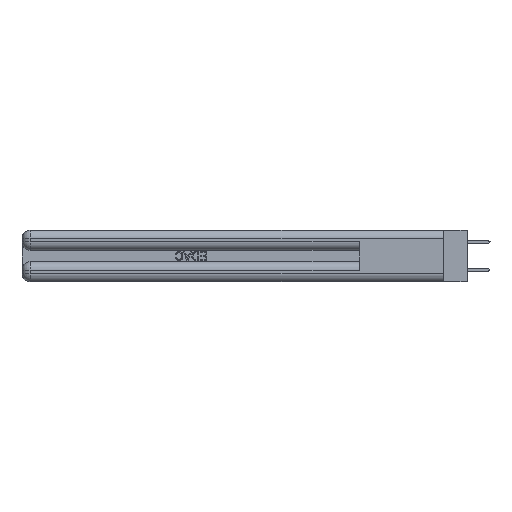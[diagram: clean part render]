
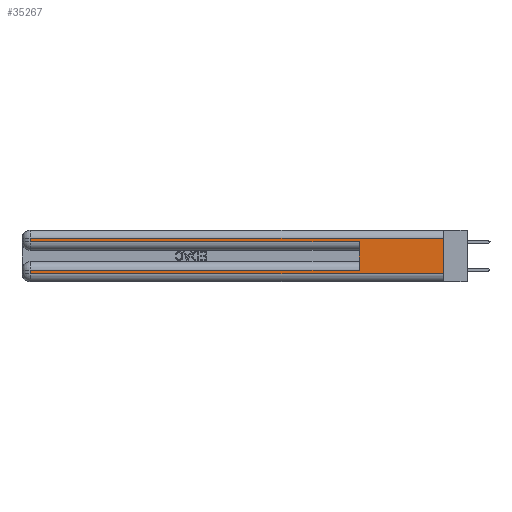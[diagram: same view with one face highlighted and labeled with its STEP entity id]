
A CAD part, left-side view. The second image highlights one B-rep face of the part: STEP entity #35267.
In plain terms, the highlighted planar face has unit normal (-1, 0, 0).
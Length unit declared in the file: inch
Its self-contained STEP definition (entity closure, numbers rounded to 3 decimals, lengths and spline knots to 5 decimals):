
#135 = ORIENTED_EDGE ( 'NONE', *, *, #6868, .T. ) ;
#209 = DIRECTION ( 'NONE',  ( 0., 1., 0. ) ) ;
#289 = CARTESIAN_POINT ( 'NONE',  ( 0., 0., 0.31 ) ) ;
#968 = VECTOR ( 'NONE', #209, 39.37008 ) ;
#1395 = LINE ( 'NONE', #9236, #25498 ) ;
#1719 = LINE ( 'NONE', #32343, #16856 ) ;
#1926 = LINE ( 'NONE', #24377, #968 ) ;
#2803 = VECTOR ( 'NONE', #30012, 39.37008 ) ;
#4164 = CARTESIAN_POINT ( 'NONE',  ( 0., 0., 0.06 ) ) ;
#4578 = CARTESIAN_POINT ( 'NONE',  ( 0., 2.94, 0.31 ) ) ;
#4890 = CARTESIAN_POINT ( 'NONE',  ( 0., 0., 0.37 ) ) ;
#5963 = CARTESIAN_POINT ( 'NONE',  ( 0., 0.6, 0.085 ) ) ;
#6315 = ORIENTED_EDGE ( 'NONE', *, *, #35557, .T. ) ;
#6868 = EDGE_CURVE ( 'NONE', #13591, #37456, #1926, .T. ) ;
#7078 = VECTOR ( 'NONE', #18430, 39.37008 ) ;
#7942 = PLANE ( 'NONE',  #19348 ) ;
#8632 = VECTOR ( 'NONE', #34360, 39.37008 ) ;
#9236 = CARTESIAN_POINT ( 'NONE',  ( 0., 2.94, 0.37 ) ) ;
#9917 = LINE ( 'NONE', #15389, #7078 ) ;
#9957 = FACE_OUTER_BOUND ( 'NONE', #37861, .T. ) ;
#10875 = LINE ( 'NONE', #24101, #2803 ) ;
#10936 = EDGE_CURVE ( 'NONE', #37456, #20333, #11874, .T. ) ;
#10943 = VECTOR ( 'NONE', #12433, 39.37008 ) ;
#11874 = LINE ( 'NONE', #27427, #10943 ) ;
#12265 = DIRECTION ( 'NONE',  ( 0., 0., -1. ) ) ;
#12402 = VECTOR ( 'NONE', #21755, 39.37008 ) ;
#12433 = DIRECTION ( 'NONE',  ( 0., 0., -1. ) ) ;
#12464 = ORIENTED_EDGE ( 'NONE', *, *, #17266, .F. ) ;
#12747 = VERTEX_POINT ( 'NONE', #4578 ) ;
#13591 = VERTEX_POINT ( 'NONE', #5963 ) ;
#14005 = DIRECTION ( 'NONE',  ( 1., 0., 0. ) ) ;
#14352 = ORIENTED_EDGE ( 'NONE', *, *, #27515, .T. ) ;
#14468 = CARTESIAN_POINT ( 'NONE',  ( 0., 2.94, 0.06 ) ) ;
#15389 = CARTESIAN_POINT ( 'NONE',  ( 0., 0., 0.285 ) ) ;
#16207 = ORIENTED_EDGE ( 'NONE', *, *, #10936, .T. ) ;
#16856 = VECTOR ( 'NONE', #29330, 39.37008 ) ;
#17266 = EDGE_CURVE ( 'NONE', #28186, #18667, #28405, .T. ) ;
#18430 = DIRECTION ( 'NONE',  ( 0., -1., 0. ) ) ;
#18501 = LINE ( 'NONE', #31327, #8632 ) ;
#18667 = VERTEX_POINT ( 'NONE', #4164 ) ;
#18722 = CARTESIAN_POINT ( 'NONE',  ( 0., 0., 0.37 ) ) ;
#19348 = AXIS2_PLACEMENT_3D ( 'NONE', #4890, #14005, #35014 ) ;
#20317 = EDGE_CURVE ( 'NONE', #20333, #18667, #1719, .T. ) ;
#20333 = VERTEX_POINT ( 'NONE', #14468 ) ;
#20448 = ORIENTED_EDGE ( 'NONE', *, *, #24747, .T. ) ;
#21755 = DIRECTION ( 'NONE',  ( 0., 0., -1. ) ) ;
#21944 = VERTEX_POINT ( 'NONE', #22452 ) ;
#22452 = CARTESIAN_POINT ( 'NONE',  ( 0., 2.94, 0.285 ) ) ;
#24101 = CARTESIAN_POINT ( 'NONE',  ( 0., 0.6, 0.145 ) ) ;
#24346 = CARTESIAN_POINT ( 'NONE',  ( 0., 2.94, 0.085 ) ) ;
#24377 = CARTESIAN_POINT ( 'NONE',  ( 0., 0., 0.085 ) ) ;
#24747 = EDGE_CURVE ( 'NONE', #28186, #12747, #18501, .T. ) ;
#25498 = VECTOR ( 'NONE', #12265, 39.37008 ) ;
#27413 = EDGE_CURVE ( 'NONE', #13591, #29452, #10875, .T. ) ;
#27427 = CARTESIAN_POINT ( 'NONE',  ( 0., 2.94, 0.37 ) ) ;
#27515 = EDGE_CURVE ( 'NONE', #21944, #29452, #9917, .T. ) ;
#28186 = VERTEX_POINT ( 'NONE', #289 ) ;
#28405 = LINE ( 'NONE', #18722, #12402 ) ;
#29330 = DIRECTION ( 'NONE',  ( 0., -1., 0. ) ) ;
#29452 = VERTEX_POINT ( 'NONE', #37052 ) ;
#30012 = DIRECTION ( 'NONE',  ( 0., 0., 1. ) ) ;
#31269 = ORIENTED_EDGE ( 'NONE', *, *, #27413, .F. ) ;
#31327 = CARTESIAN_POINT ( 'NONE',  ( 0., 0., 0.31 ) ) ;
#32343 = CARTESIAN_POINT ( 'NONE',  ( 0., 0., 0.06 ) ) ;
#34093 = ORIENTED_EDGE ( 'NONE', *, *, #20317, .T. ) ;
#34360 = DIRECTION ( 'NONE',  ( 0., 1., 0. ) ) ;
#35014 = DIRECTION ( 'NONE',  ( 0., 0., -1. ) ) ;
#35267 = ADVANCED_FACE ( 'NONE', ( #9957 ), #7942, .F. ) ;
#35557 = EDGE_CURVE ( 'NONE', #12747, #21944, #1395, .T. ) ;
#37052 = CARTESIAN_POINT ( 'NONE',  ( 0., 0.6, 0.285 ) ) ;
#37456 = VERTEX_POINT ( 'NONE', #24346 ) ;
#37861 = EDGE_LOOP ( 'NONE', ( #12464, #20448, #6315, #14352, #31269, #135, #16207, #34093 ) ) ;
